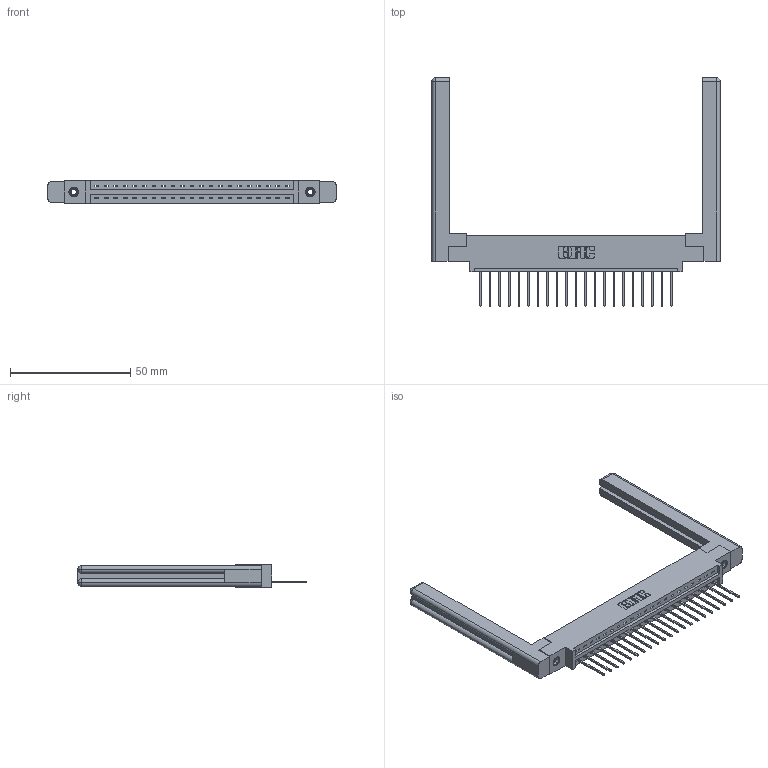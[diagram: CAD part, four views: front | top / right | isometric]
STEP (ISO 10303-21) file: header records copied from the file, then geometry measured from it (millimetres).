
FILE_DESCRIPTION (( 'STEP AP203' ), '1' );
FILE_NAME ('337-021-540-658.STEP', '2019-09-29T00:40:23', ( '' ), ( '' ), 'SwSTEP 2.0', 'SolidWorks 2016', '' );
FILE_SCHEMA (( 'CONFIG_CONTROL_DESIGN' ));
Length unit declared in the file: inch
Products named in the file (5): 337-021-540-658; 307-220-058; 345-292-001_345-293-140; 337 Part_0.170 Offset - 0.156 Dia-TI; 345-250-001_345-250-001-102
Assembly tree (26 placements, depth 2):
  337-021-540-658
    337 Part_0.170 Offset - 0.156 Dia-TI
    345-292-001_345-293-140  x21
    345-250-001_345-250-001-102  x2
    307-220-058  x2
Bounding box: 119.84 x 94.87 x 9.4 mm (x, y, z)
Volume: 19265.4 mm3; surface area: 17910.8 mm2
Topology: 26 solids, 26 shells, 1562 faces, 4625 edges, 3042 vertices
Faces by surface type: plane 1124, cylinder 414, cone 12, torus 12
Entity records: 21110 total; most frequent: CARTESIAN_POINT 3676, ORIENTED_EDGE 3572, DIRECTION 3156, EDGE_CURVE 1786, LINE 1610, VECTOR 1610, VERTEX_POINT 1182, AXIS2_PLACEMENT_3D 773
